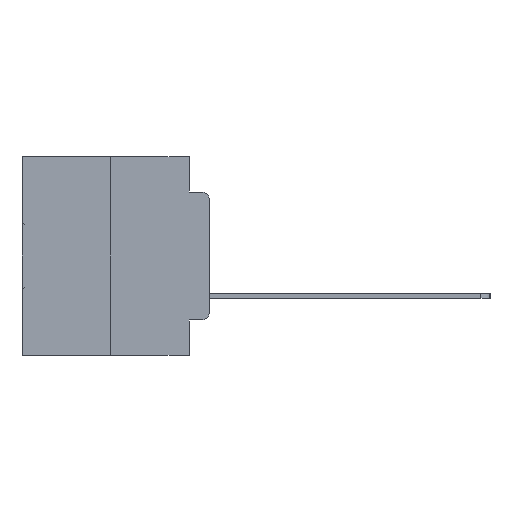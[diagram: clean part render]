
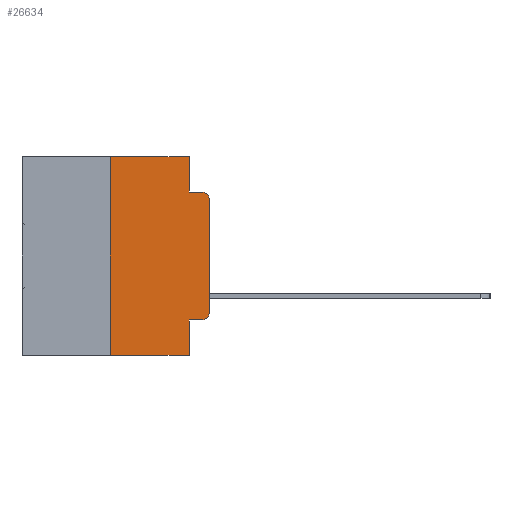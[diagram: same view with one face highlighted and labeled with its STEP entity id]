
A CAD part, left-side view. The second image highlights one B-rep face of the part: STEP entity #26634.
In plain terms, the highlighted planar face has unit normal (-1, 0, 0).
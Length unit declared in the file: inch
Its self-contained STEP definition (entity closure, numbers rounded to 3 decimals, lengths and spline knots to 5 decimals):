
#230 = EDGE_CURVE ( 'NONE', #27326, #16782, #30859, .T. ) ;
#754 = CARTESIAN_POINT ( 'NONE',  ( 0., 0.25, -0.5 ) ) ;
#765 = VECTOR ( 'NONE', #17539, 39.37008 ) ;
#832 = VERTEX_POINT ( 'NONE', #10803 ) ;
#1034 = ORIENTED_EDGE ( 'NONE', *, *, #2559, .T. ) ;
#1776 = DIRECTION ( 'NONE',  ( 0., -1., 0. ) ) ;
#2144 = VECTOR ( 'NONE', #25331, 39.37008 ) ;
#2382 = DIRECTION ( 'NONE',  ( 0., -1., 0. ) ) ;
#2559 = EDGE_CURVE ( 'NONE', #27807, #16782, #32113, .T. ) ;
#3061 = LINE ( 'NONE', #29350, #22356 ) ;
#3536 = VECTOR ( 'NONE', #19245, 39.37008 ) ;
#3584 = EDGE_CURVE ( 'NONE', #12628, #17507, #3061, .T. ) ;
#4616 = LINE ( 'NONE', #7641, #15669 ) ;
#5696 = CARTESIAN_POINT ( 'NONE',  ( 0., 0.051, -0.0885 ) ) ;
#5965 = DIRECTION ( 'NONE',  ( -1., 0., 0. ) ) ;
#6172 = EDGE_CURVE ( 'NONE', #27807, #832, #14778, .T. ) ;
#7337 = EDGE_CURVE ( 'NONE', #10666, #17507, #30310, .T. ) ;
#7498 = VERTEX_POINT ( 'NONE', #18366 ) ;
#7641 = CARTESIAN_POINT ( 'NONE',  ( 0., 0.473, 0. ) ) ;
#8369 = LINE ( 'NONE', #15013, #765 ) ;
#8439 = DIRECTION ( 'NONE',  ( 0., 0., -1. ) ) ;
#8623 = FACE_OUTER_BOUND ( 'NONE', #10625, .T. ) ;
#9422 = ORIENTED_EDGE ( 'NONE', *, *, #230, .F. ) ;
#9574 = EDGE_CURVE ( 'NONE', #832, #18634, #4616, .T. ) ;
#10136 = CARTESIAN_POINT ( 'NONE',  ( 0., 0., -0.1085 ) ) ;
#10278 = LINE ( 'NONE', #26685, #3536 ) ;
#10348 = CARTESIAN_POINT ( 'NONE',  ( 0., 0.25, 0. ) ) ;
#10625 = EDGE_LOOP ( 'NONE', ( #27123, #19860, #23815, #12907, #28194, #17235, #1034, #9422, #22751, #11766 ) ) ;
#10666 = VERTEX_POINT ( 'NONE', #10136 ) ;
#10803 = CARTESIAN_POINT ( 'NONE',  ( 0., 0.25, 0. ) ) ;
#10983 = VECTOR ( 'NONE', #17418, 39.37008 ) ;
#11766 = ORIENTED_EDGE ( 'NONE', *, *, #21754, .T. ) ;
#12448 = CARTESIAN_POINT ( 'NONE',  ( 0., 0.473, -0.5 ) ) ;
#12628 = VERTEX_POINT ( 'NONE', #5696 ) ;
#12702 = CARTESIAN_POINT ( 'NONE',  ( 0., 0.473, 0. ) ) ;
#12796 = DIRECTION ( 'NONE',  ( -1., 0., 0. ) ) ;
#12907 = ORIENTED_EDGE ( 'NONE', *, *, #25244, .F. ) ;
#13407 = CARTESIAN_POINT ( 'NONE',  ( 0., 0.051, -0.5 ) ) ;
#13457 = CARTESIAN_POINT ( 'NONE',  ( 0., 0.02, -0.4115 ) ) ;
#13734 = CARTESIAN_POINT ( 'NONE',  ( 0., 0.051, 0. ) ) ;
#14778 = LINE ( 'NONE', #10348, #2144 ) ;
#15013 = CARTESIAN_POINT ( 'NONE',  ( 0., 0.051, -0.4115 ) ) ;
#15102 = PLANE ( 'NONE',  #19782 ) ;
#15220 = DIRECTION ( 'NONE',  ( 0., 0., -1. ) ) ;
#15669 = VECTOR ( 'NONE', #17723, 39.37008 ) ;
#16782 = VERTEX_POINT ( 'NONE', #13407 ) ;
#17056 = EDGE_CURVE ( 'NONE', #27326, #22449, #8369, .T. ) ;
#17077 = AXIS2_PLACEMENT_3D ( 'NONE', #27793, #12796, #30256 ) ;
#17235 = ORIENTED_EDGE ( 'NONE', *, *, #6172, .F. ) ;
#17418 = DIRECTION ( 'NONE',  ( 0., 0., 1. ) ) ;
#17507 = VERTEX_POINT ( 'NONE', #19363 ) ;
#17539 = DIRECTION ( 'NONE',  ( 0., -1., 0. ) ) ;
#17723 = DIRECTION ( 'NONE',  ( 0., -1., 0. ) ) ;
#18366 = CARTESIAN_POINT ( 'NONE',  ( 0., 0., -0.3915 ) ) ;
#18413 = LINE ( 'NONE', #32308, #10983 ) ;
#18634 = VERTEX_POINT ( 'NONE', #13734 ) ;
#19245 = DIRECTION ( 'NONE',  ( 0., 0., -1. ) ) ;
#19363 = CARTESIAN_POINT ( 'NONE',  ( 0., 0.02, -0.0885 ) ) ;
#19782 = AXIS2_PLACEMENT_3D ( 'NONE', #12702, #30159, #15220 ) ;
#19860 = ORIENTED_EDGE ( 'NONE', *, *, #7337, .T. ) ;
#20445 = CARTESIAN_POINT ( 'NONE',  ( 0., 0.051, -0.4115 ) ) ;
#20927 = CARTESIAN_POINT ( 'NONE',  ( 0., 0.051, 0. ) ) ;
#21028 = CARTESIAN_POINT ( 'NONE',  ( 0., 0.02, -0.3915 ) ) ;
#21754 = EDGE_CURVE ( 'NONE', #22449, #7498, #29675, .T. ) ;
#22356 = VECTOR ( 'NONE', #1776, 39.37008 ) ;
#22449 = VERTEX_POINT ( 'NONE', #13457 ) ;
#22751 = ORIENTED_EDGE ( 'NONE', *, *, #17056, .T. ) ;
#23551 = DIRECTION ( 'NONE',  ( 0., 0., -1. ) ) ;
#23697 = AXIS2_PLACEMENT_3D ( 'NONE', #21028, #5965, #23551 ) ;
#23815 = ORIENTED_EDGE ( 'NONE', *, *, #3584, .F. ) ;
#25244 = EDGE_CURVE ( 'NONE', #18634, #12628, #10278, .T. ) ;
#25331 = DIRECTION ( 'NONE',  ( 0., 0., 1. ) ) ;
#25548 = VECTOR ( 'NONE', #2382, 39.37008 ) ;
#26549 = EDGE_CURVE ( 'NONE', #7498, #10666, #18413, .T. ) ;
#26634 = ADVANCED_FACE ( 'NONE', ( #8623 ), #15102, .F. ) ;
#26685 = CARTESIAN_POINT ( 'NONE',  ( 0., 0.051, 0. ) ) ;
#27123 = ORIENTED_EDGE ( 'NONE', *, *, #26549, .T. ) ;
#27326 = VERTEX_POINT ( 'NONE', #20445 ) ;
#27793 = CARTESIAN_POINT ( 'NONE',  ( 0., 0.02, -0.1085 ) ) ;
#27807 = VERTEX_POINT ( 'NONE', #754 ) ;
#28194 = ORIENTED_EDGE ( 'NONE', *, *, #9574, .F. ) ;
#29350 = CARTESIAN_POINT ( 'NONE',  ( 0., 0.051, -0.0885 ) ) ;
#29675 = CIRCLE ( 'NONE', #23697, 0.02 ) ;
#30076 = VECTOR ( 'NONE', #8439, 39.37008 ) ;
#30159 = DIRECTION ( 'NONE',  ( 1., 0., 0. ) ) ;
#30256 = DIRECTION ( 'NONE',  ( 0., 0., -1. ) ) ;
#30310 = CIRCLE ( 'NONE', #17077, 0.02 ) ;
#30859 = LINE ( 'NONE', #20927, #30076 ) ;
#32113 = LINE ( 'NONE', #12448, #25548 ) ;
#32308 = CARTESIAN_POINT ( 'NONE',  ( 0., 0., 0. ) ) ;
